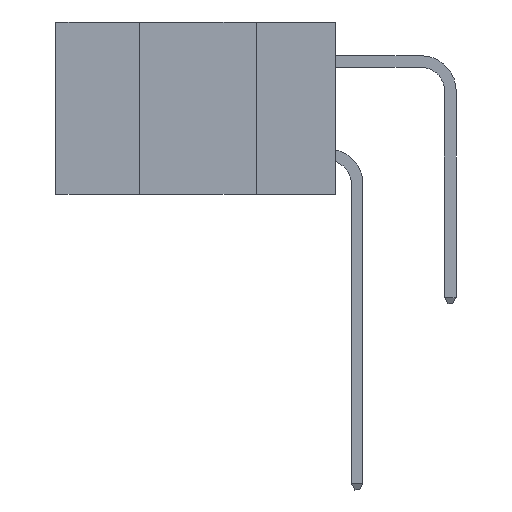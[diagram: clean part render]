
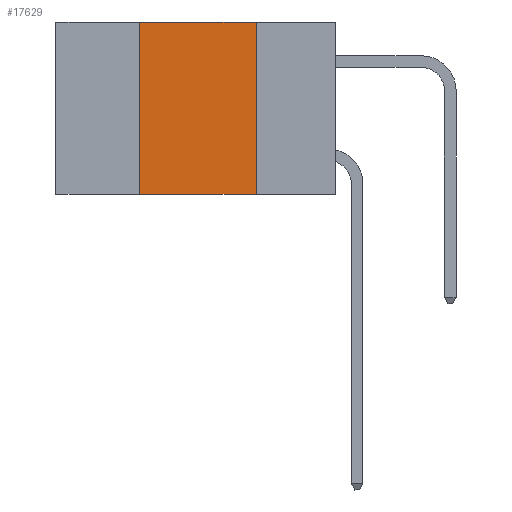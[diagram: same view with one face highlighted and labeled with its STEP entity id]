
A CAD part, left-side view. The second image highlights one B-rep face of the part: STEP entity #17629.
In plain terms, the highlighted planar face has unit normal (-1, 0, 0).
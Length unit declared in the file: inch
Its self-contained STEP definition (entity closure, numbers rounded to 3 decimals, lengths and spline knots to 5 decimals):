
#868 = LINE ( 'NONE', #12036, #6465 ) ;
#952 = ORIENTED_EDGE ( 'NONE', *, *, #1041, .T. ) ;
#1041 = EDGE_CURVE ( 'NONE', #6954, #8148, #868, .T. ) ;
#1110 = EDGE_CURVE ( 'NONE', #8613, #1405, #1962, .T. ) ;
#1405 = VERTEX_POINT ( 'NONE', #8351 ) ;
#1445 = CARTESIAN_POINT ( 'NONE',  ( 0., 0.6, 0. ) ) ;
#1523 = VECTOR ( 'NONE', #8205, 39.37008 ) ;
#1962 = LINE ( 'NONE', #8147, #1523 ) ;
#3599 = LINE ( 'NONE', #17051, #16142 ) ;
#4875 = ORIENTED_EDGE ( 'NONE', *, *, #18278, .F. ) ;
#5500 = DIRECTION ( 'NONE',  ( 0., 0., -1. ) ) ;
#5996 = CARTESIAN_POINT ( 'NONE',  ( 0., 0.17, 0. ) ) ;
#6141 = ORIENTED_EDGE ( 'NONE', *, *, #1110, .F. ) ;
#6465 = VECTOR ( 'NONE', #14046, 39.37008 ) ;
#6954 = VERTEX_POINT ( 'NONE', #11948 ) ;
#7264 = CARTESIAN_POINT ( 'NONE',  ( 0., 0.17, -0.37 ) ) ;
#8147 = CARTESIAN_POINT ( 'NONE',  ( 0., 0.6, 0. ) ) ;
#8148 = VERTEX_POINT ( 'NONE', #7264 ) ;
#8205 = DIRECTION ( 'NONE',  ( 0., -1., 0. ) ) ;
#8351 = CARTESIAN_POINT ( 'NONE',  ( 0., 0.17, 0. ) ) ;
#8613 = VERTEX_POINT ( 'NONE', #13257 ) ;
#8652 = EDGE_LOOP ( 'NONE', ( #4875, #6141, #14548, #952 ) ) ;
#8870 = DIRECTION ( 'NONE',  ( 0., 0., -1. ) ) ;
#8974 = FACE_OUTER_BOUND ( 'NONE', #8652, .T. ) ;
#9937 = PLANE ( 'NONE',  #13110 ) ;
#11948 = CARTESIAN_POINT ( 'NONE',  ( 0., 0.42, -0.37 ) ) ;
#12036 = CARTESIAN_POINT ( 'NONE',  ( 0., 0.6, -0.37 ) ) ;
#12303 = LINE ( 'NONE', #5996, #13421 ) ;
#12772 = DIRECTION ( 'NONE',  ( 0., 0., 1. ) ) ;
#13110 = AXIS2_PLACEMENT_3D ( 'NONE', #1445, #15767, #5500 ) ;
#13257 = CARTESIAN_POINT ( 'NONE',  ( 0., 0.42, 0. ) ) ;
#13421 = VECTOR ( 'NONE', #8870, 39.37008 ) ;
#14046 = DIRECTION ( 'NONE',  ( 0., -1., 0. ) ) ;
#14414 = EDGE_CURVE ( 'NONE', #6954, #8613, #3599, .T. ) ;
#14548 = ORIENTED_EDGE ( 'NONE', *, *, #14414, .F. ) ;
#15767 = DIRECTION ( 'NONE',  ( 1., 0., 0. ) ) ;
#16142 = VECTOR ( 'NONE', #12772, 39.37008 ) ;
#17051 = CARTESIAN_POINT ( 'NONE',  ( 0., 0.42, 0. ) ) ;
#17629 = ADVANCED_FACE ( 'NONE', ( #8974 ), #9937, .F. ) ;
#18278 = EDGE_CURVE ( 'NONE', #1405, #8148, #12303, .T. ) ;
